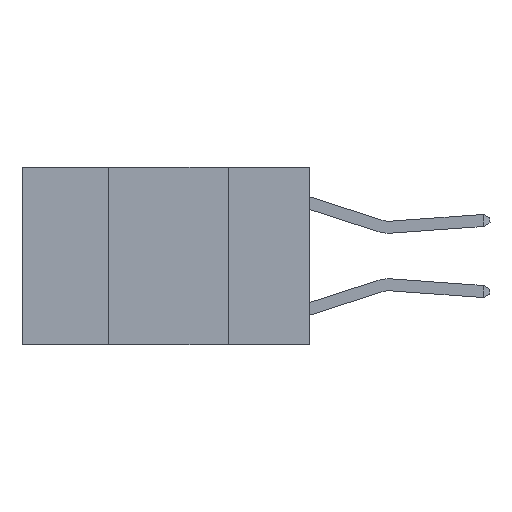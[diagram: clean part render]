
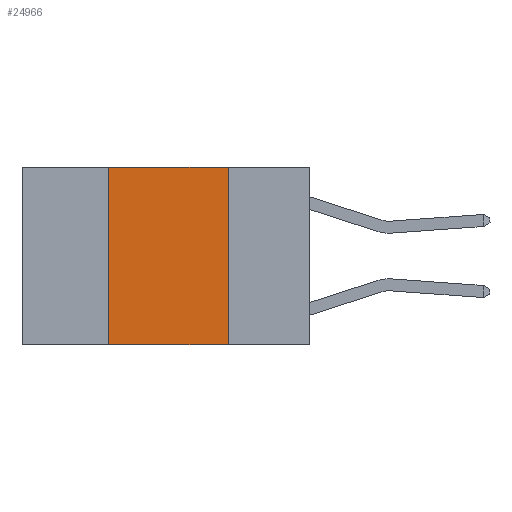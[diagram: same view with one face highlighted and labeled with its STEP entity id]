
A CAD part, left-side view. The second image highlights one B-rep face of the part: STEP entity #24966.
In plain terms, the highlighted planar face has unit normal (-1, 0, 0).
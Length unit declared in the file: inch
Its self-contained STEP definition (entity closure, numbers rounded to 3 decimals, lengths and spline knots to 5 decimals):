
#304 = EDGE_CURVE ( 'NONE', #14251, #29040, #7373, .T. ) ;
#852 = DIRECTION ( 'NONE',  ( 0., -1., 0. ) ) ;
#1913 = VECTOR ( 'NONE', #20957, 39.37008 ) ;
#2394 = VECTOR ( 'NONE', #852, 39.37008 ) ;
#3407 = LINE ( 'NONE', #8962, #1913 ) ;
#6340 = ORIENTED_EDGE ( 'NONE', *, *, #10671, .F. ) ;
#6715 = AXIS2_PLACEMENT_3D ( 'NONE', #21030, #25991, #11467 ) ;
#7074 = ORIENTED_EDGE ( 'NONE', *, *, #25362, .F. ) ;
#7373 = LINE ( 'NONE', #30971, #26004 ) ;
#8001 = DIRECTION ( 'NONE',  ( 0., 0., -1. ) ) ;
#8962 = CARTESIAN_POINT ( 'NONE',  ( 0., 0.42, 0. ) ) ;
#10118 = EDGE_CURVE ( 'NONE', #11062, #29040, #18824, .T. ) ;
#10671 = EDGE_CURVE ( 'NONE', #18781, #11062, #28267, .T. ) ;
#11062 = VERTEX_POINT ( 'NONE', #16690 ) ;
#11467 = DIRECTION ( 'NONE',  ( 0., 0., -1. ) ) ;
#11592 = DIRECTION ( 'NONE',  ( 0., -1., 0. ) ) ;
#12504 = EDGE_LOOP ( 'NONE', ( #17753, #6340, #7074, #13590 ) ) ;
#12800 = CARTESIAN_POINT ( 'NONE',  ( 0., 0.17, 0. ) ) ;
#12991 = CARTESIAN_POINT ( 'NONE',  ( 0., 0.6, 0. ) ) ;
#13118 = VECTOR ( 'NONE', #8001, 39.37008 ) ;
#13590 = ORIENTED_EDGE ( 'NONE', *, *, #304, .T. ) ;
#13829 = PLANE ( 'NONE',  #6715 ) ;
#14251 = VERTEX_POINT ( 'NONE', #14314 ) ;
#14314 = CARTESIAN_POINT ( 'NONE',  ( 0., 0.42, -0.37 ) ) ;
#16690 = CARTESIAN_POINT ( 'NONE',  ( 0., 0.17, 0. ) ) ;
#17753 = ORIENTED_EDGE ( 'NONE', *, *, #10118, .F. ) ;
#18781 = VERTEX_POINT ( 'NONE', #30564 ) ;
#18824 = LINE ( 'NONE', #12800, #13118 ) ;
#19798 = FACE_OUTER_BOUND ( 'NONE', #12504, .T. ) ;
#20957 = DIRECTION ( 'NONE',  ( 0., 0., 1. ) ) ;
#21030 = CARTESIAN_POINT ( 'NONE',  ( 0., 0.6, 0. ) ) ;
#22686 = CARTESIAN_POINT ( 'NONE',  ( 0., 0.17, -0.37 ) ) ;
#24966 = ADVANCED_FACE ( 'NONE', ( #19798 ), #13829, .F. ) ;
#25362 = EDGE_CURVE ( 'NONE', #14251, #18781, #3407, .T. ) ;
#25991 = DIRECTION ( 'NONE',  ( 1., 0., 0. ) ) ;
#26004 = VECTOR ( 'NONE', #11592, 39.37008 ) ;
#28267 = LINE ( 'NONE', #12991, #2394 ) ;
#29040 = VERTEX_POINT ( 'NONE', #22686 ) ;
#30564 = CARTESIAN_POINT ( 'NONE',  ( 0., 0.42, 0. ) ) ;
#30971 = CARTESIAN_POINT ( 'NONE',  ( 0., 0.6, -0.37 ) ) ;
